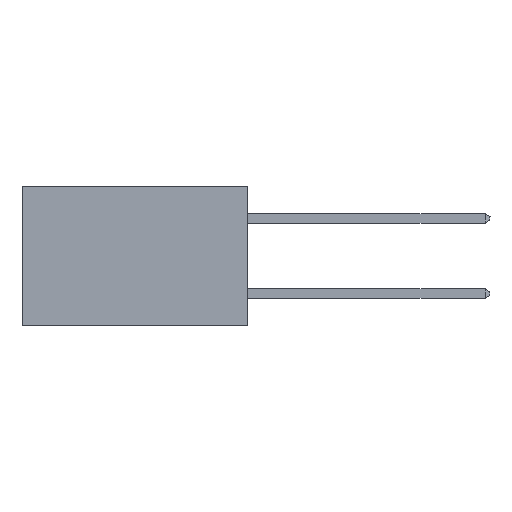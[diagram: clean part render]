
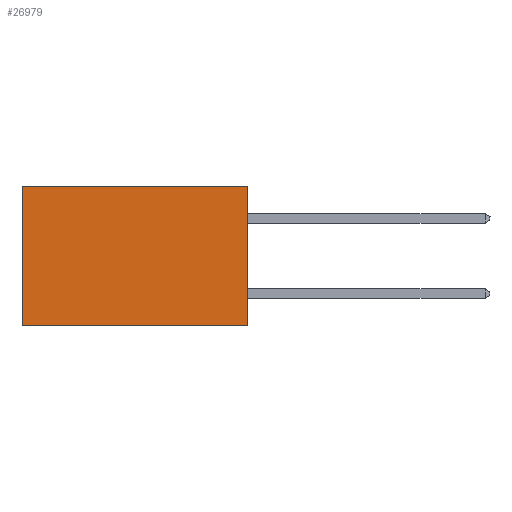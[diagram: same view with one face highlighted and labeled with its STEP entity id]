
A CAD part, left-side view. The second image highlights one B-rep face of the part: STEP entity #26979.
In plain terms, the highlighted planar face has unit normal (-1, 0, 0).
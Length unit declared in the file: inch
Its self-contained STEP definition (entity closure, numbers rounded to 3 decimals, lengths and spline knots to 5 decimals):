
#131 = CARTESIAN_POINT ( 'NONE',  ( 0.298, 0., 0. ) ) ;
#238 = DIRECTION ( 'NONE',  ( 0., 0., -1. ) ) ;
#880 = VERTEX_POINT ( 'NONE', #29045 ) ;
#1979 = DIRECTION ( 'NONE',  ( 0., 0., -1. ) ) ;
#4347 = LINE ( 'NONE', #7275, #17023 ) ;
#5205 = AXIS2_PLACEMENT_3D ( 'NONE', #31850, #17176, #1979 ) ;
#6273 = VECTOR ( 'NONE', #10224, 39.37008 ) ;
#7268 = EDGE_LOOP ( 'NONE', ( #29314, #27127, #26969, #14768 ) ) ;
#7275 = CARTESIAN_POINT ( 'NONE',  ( 0.298, 0., -0.37 ) ) ;
#9148 = VERTEX_POINT ( 'NONE', #23091 ) ;
#9826 = DIRECTION ( 'NONE',  ( 0., 1., 0. ) ) ;
#10224 = DIRECTION ( 'NONE',  ( 0., 1., 0. ) ) ;
#11053 = VECTOR ( 'NONE', #25470, 39.37008 ) ;
#11152 = VECTOR ( 'NONE', #238, 39.37008 ) ;
#13981 = VERTEX_POINT ( 'NONE', #16462 ) ;
#14768 = ORIENTED_EDGE ( 'NONE', *, *, #27114, .T. ) ;
#16462 = CARTESIAN_POINT ( 'NONE',  ( 0.298, 0., 0. ) ) ;
#17023 = VECTOR ( 'NONE', #9826, 39.37008 ) ;
#17176 = DIRECTION ( 'NONE',  ( 1., 0., 0. ) ) ;
#17863 = LINE ( 'NONE', #131, #11152 ) ;
#18814 = EDGE_CURVE ( 'NONE', #25383, #9148, #4347, .T. ) ;
#22731 = CARTESIAN_POINT ( 'NONE',  ( 0.298, 0., 0. ) ) ;
#23021 = CARTESIAN_POINT ( 'NONE',  ( 0.298, 0.6, 0. ) ) ;
#23091 = CARTESIAN_POINT ( 'NONE',  ( 0.298, 0.6, -0.37 ) ) ;
#24369 = LINE ( 'NONE', #23021, #11053 ) ;
#24560 = PLANE ( 'NONE',  #5205 ) ;
#24603 = EDGE_CURVE ( 'NONE', #13981, #25383, #17863, .T. ) ;
#25383 = VERTEX_POINT ( 'NONE', #28067 ) ;
#25470 = DIRECTION ( 'NONE',  ( 0., 0., -1. ) ) ;
#25888 = EDGE_CURVE ( 'NONE', #880, #9148, #24369, .T. ) ;
#26230 = LINE ( 'NONE', #22731, #6273 ) ;
#26969 = ORIENTED_EDGE ( 'NONE', *, *, #24603, .F. ) ;
#26979 = ADVANCED_FACE ( 'NONE', ( #30053 ), #24560, .F. ) ;
#27114 = EDGE_CURVE ( 'NONE', #13981, #880, #26230, .T. ) ;
#27127 = ORIENTED_EDGE ( 'NONE', *, *, #18814, .F. ) ;
#28067 = CARTESIAN_POINT ( 'NONE',  ( 0.298, 0., -0.37 ) ) ;
#29045 = CARTESIAN_POINT ( 'NONE',  ( 0.298, 0.6, 0. ) ) ;
#29314 = ORIENTED_EDGE ( 'NONE', *, *, #25888, .T. ) ;
#30053 = FACE_OUTER_BOUND ( 'NONE', #7268, .T. ) ;
#31850 = CARTESIAN_POINT ( 'NONE',  ( 0.298, 0., 0. ) ) ;
